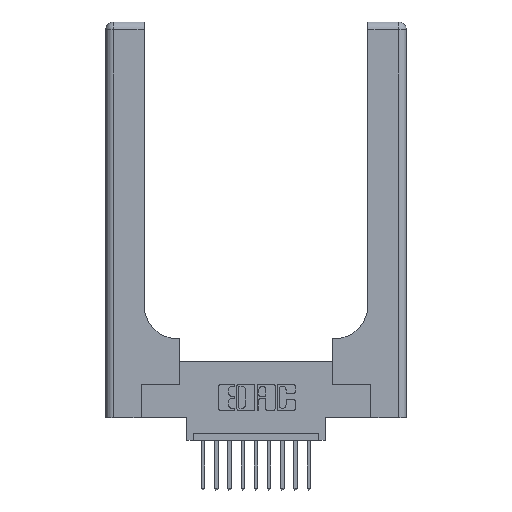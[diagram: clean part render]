
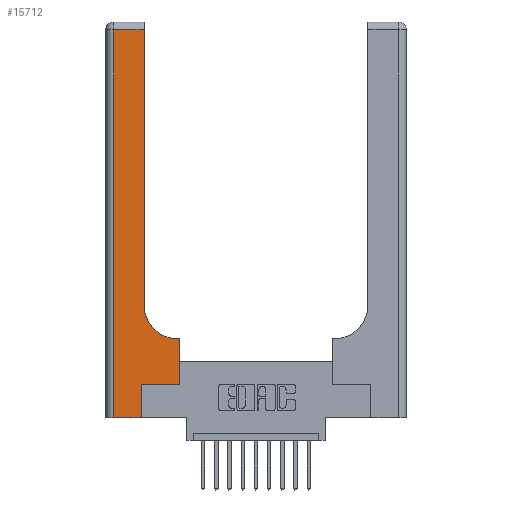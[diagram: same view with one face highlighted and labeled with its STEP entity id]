
A CAD part, top view. The second image highlights one B-rep face of the part: STEP entity #15712.
In plain terms, the highlighted planar face has unit normal (0, 0, 1).
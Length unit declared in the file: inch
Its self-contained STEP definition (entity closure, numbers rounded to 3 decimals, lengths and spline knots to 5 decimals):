
#511 = DIRECTION ( 'NONE',  ( 0., 0., -1. ) ) ;
#594 = AXIS2_PLACEMENT_3D ( 'NONE', #738, #511, #6931 ) ;
#680 = DIRECTION ( 'NONE',  ( 0., 1., 0. ) ) ;
#711 = ORIENTED_EDGE ( 'NONE', *, *, #15640, .T. ) ;
#738 = CARTESIAN_POINT ( 'NONE',  ( 0., 3., 0.37 ) ) ;
#861 = VERTEX_POINT ( 'NONE', #2688 ) ;
#1058 = DIRECTION ( 'NONE',  ( -1., 0., 0. ) ) ;
#1333 = VECTOR ( 'NONE', #15839, 39.37008 ) ;
#1563 = EDGE_CURVE ( 'NONE', #7000, #7262, #9719, .T. ) ;
#2047 = CARTESIAN_POINT ( 'NONE',  ( 0.2915, 0.85, 0.37 ) ) ;
#2180 = CARTESIAN_POINT ( 'NONE',  ( 0.2915, 3., 0.37 ) ) ;
#2369 = CARTESIAN_POINT ( 'NONE',  ( 0.5585, 0.25, 0.37 ) ) ;
#2426 = CARTESIAN_POINT ( 'NONE',  ( 0.269, 0., 0.37 ) ) ;
#2688 = CARTESIAN_POINT ( 'NONE',  ( 0.06, 2.94, 0.37 ) ) ;
#2713 = CARTESIAN_POINT ( 'NONE',  ( 0.5585, 0.25, 0.37 ) ) ;
#3204 = DIRECTION ( 'NONE',  ( 0., 0., -1. ) ) ;
#3250 = LINE ( 'NONE', #2713, #15817 ) ;
#3396 = CARTESIAN_POINT ( 'NONE',  ( 0.2915, 2.94, 0.37 ) ) ;
#3634 = LINE ( 'NONE', #7043, #5398 ) ;
#4085 = DIRECTION ( 'NONE',  ( 0., -1., 0. ) ) ;
#4119 = VECTOR ( 'NONE', #10908, 39.37008 ) ;
#4588 = EDGE_CURVE ( 'NONE', #16576, #8240, #3250, .T. ) ;
#5398 = VECTOR ( 'NONE', #8437, 39.37008 ) ;
#5452 = CARTESIAN_POINT ( 'NONE',  ( 0.06, 3., 0.37 ) ) ;
#5462 = VERTEX_POINT ( 'NONE', #3396 ) ;
#5526 = CARTESIAN_POINT ( 'NONE',  ( 0.269, 0.25, 0.37 ) ) ;
#5672 = ORIENTED_EDGE ( 'NONE', *, *, #7364, .T. ) ;
#5745 = CARTESIAN_POINT ( 'NONE',  ( 0.5415, 0.85, 0.37 ) ) ;
#5776 = CARTESIAN_POINT ( 'NONE',  ( 0.5585, 0.6, 0.37 ) ) ;
#5903 = DIRECTION ( 'NONE',  ( 0., 1., 0. ) ) ;
#6502 = LINE ( 'NONE', #10795, #4119 ) ;
#6804 = CARTESIAN_POINT ( 'NONE',  ( 0.5415, 0.6, 0.37 ) ) ;
#6928 = VERTEX_POINT ( 'NONE', #2426 ) ;
#6931 = DIRECTION ( 'NONE',  ( -1., 0., 0. ) ) ;
#7000 = VERTEX_POINT ( 'NONE', #6804 ) ;
#7043 = CARTESIAN_POINT ( 'NONE',  ( 0., 0., 0.37 ) ) ;
#7262 = VERTEX_POINT ( 'NONE', #2047 ) ;
#7346 = VECTOR ( 'NONE', #4085, 39.37008 ) ;
#7364 = EDGE_CURVE ( 'NONE', #13550, #6928, #3634, .T. ) ;
#8240 = VERTEX_POINT ( 'NONE', #5776 ) ;
#8437 = DIRECTION ( 'NONE',  ( 1., 0., 0. ) ) ;
#8488 = CARTESIAN_POINT ( 'NONE',  ( 0.269, 0., 0.37 ) ) ;
#8575 = VECTOR ( 'NONE', #680, 39.37008 ) ;
#9129 = LINE ( 'NONE', #5452, #7346 ) ;
#9719 = CIRCLE ( 'NONE', #9731, 0.25 ) ;
#9731 = AXIS2_PLACEMENT_3D ( 'NONE', #5745, #3204, #10960 ) ;
#10012 = EDGE_CURVE ( 'NONE', #5462, #861, #12328, .T. ) ;
#10299 = ORIENTED_EDGE ( 'NONE', *, *, #10012, .T. ) ;
#10302 = VECTOR ( 'NONE', #5903, 39.37008 ) ;
#10771 = LINE ( 'NONE', #8488, #8575 ) ;
#10795 = CARTESIAN_POINT ( 'NONE',  ( 0.269, 0.25, 0.37 ) ) ;
#10908 = DIRECTION ( 'NONE',  ( 1., 0., 0. ) ) ;
#10960 = DIRECTION ( 'NONE',  ( 1., 0., 0. ) ) ;
#11501 = EDGE_CURVE ( 'NONE', #11574, #16576, #6502, .T. ) ;
#11574 = VERTEX_POINT ( 'NONE', #5526 ) ;
#11820 = ORIENTED_EDGE ( 'NONE', *, *, #11501, .T. ) ;
#12120 = PLANE ( 'NONE',  #594 ) ;
#12309 = EDGE_CURVE ( 'NONE', #8240, #7000, #16087, .T. ) ;
#12328 = LINE ( 'NONE', #12847, #1333 ) ;
#12602 = ORIENTED_EDGE ( 'NONE', *, *, #1563, .T. ) ;
#12632 = CARTESIAN_POINT ( 'NONE',  ( 0.06, 0., 0.37 ) ) ;
#12847 = CARTESIAN_POINT ( 'NONE',  ( 0., 2.94, 0.37 ) ) ;
#12913 = FACE_OUTER_BOUND ( 'NONE', #15376, .T. ) ;
#13550 = VERTEX_POINT ( 'NONE', #12632 ) ;
#13653 = CARTESIAN_POINT ( 'NONE',  ( 0.2915, 0.6, 0.37 ) ) ;
#14079 = VECTOR ( 'NONE', #1058, 39.37008 ) ;
#14102 = ORIENTED_EDGE ( 'NONE', *, *, #14507, .T. ) ;
#14121 = LINE ( 'NONE', #2180, #10302 ) ;
#14263 = ORIENTED_EDGE ( 'NONE', *, *, #4588, .T. ) ;
#14379 = DIRECTION ( 'NONE',  ( 0., 1., 0. ) ) ;
#14507 = EDGE_CURVE ( 'NONE', #6928, #11574, #10771, .T. ) ;
#15376 = EDGE_LOOP ( 'NONE', ( #16241, #10299, #711, #5672, #14102, #11820, #14263, #15429, #12602 ) ) ;
#15429 = ORIENTED_EDGE ( 'NONE', *, *, #12309, .T. ) ;
#15640 = EDGE_CURVE ( 'NONE', #861, #13550, #9129, .T. ) ;
#15712 = ADVANCED_FACE ( 'NONE', ( #12913 ), #12120, .F. ) ;
#15817 = VECTOR ( 'NONE', #14379, 39.37008 ) ;
#15839 = DIRECTION ( 'NONE',  ( -1., 0., 0. ) ) ;
#15846 = EDGE_CURVE ( 'NONE', #7262, #5462, #14121, .T. ) ;
#16087 = LINE ( 'NONE', #13653, #14079 ) ;
#16241 = ORIENTED_EDGE ( 'NONE', *, *, #15846, .T. ) ;
#16576 = VERTEX_POINT ( 'NONE', #2369 ) ;
